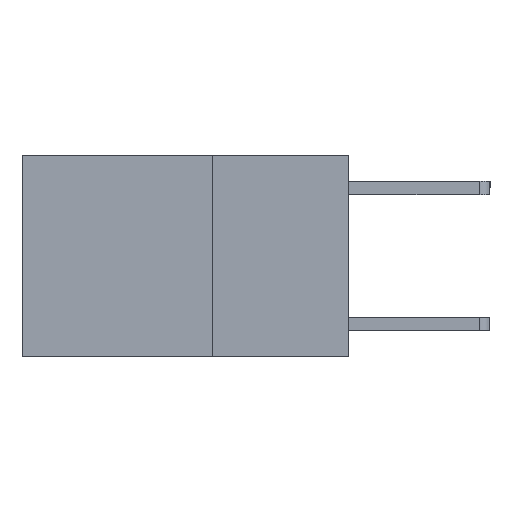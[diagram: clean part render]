
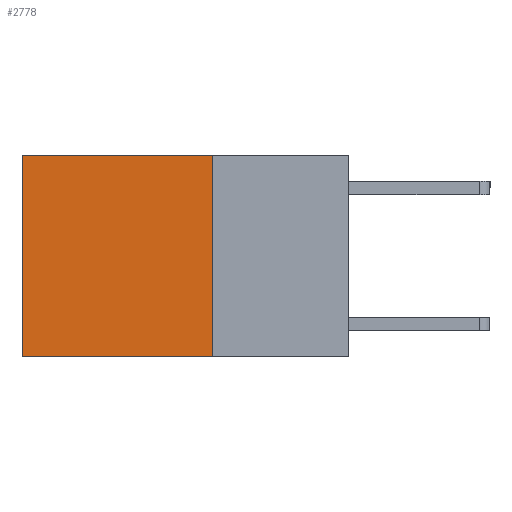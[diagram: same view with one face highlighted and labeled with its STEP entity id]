
A CAD part, left-side view. The second image highlights one B-rep face of the part: STEP entity #2778.
In plain terms, the highlighted planar face has unit normal (-1, 0, 0).
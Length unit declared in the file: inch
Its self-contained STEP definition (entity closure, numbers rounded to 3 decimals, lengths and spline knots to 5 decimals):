
#118 = VECTOR ( 'NONE', #6369, 39.37008 ) ;
#669 = VECTOR ( 'NONE', #2385, 39.37008 ) ;
#998 = AXIS2_PLACEMENT_3D ( 'NONE', #3010, #8167, #5518 ) ;
#1388 = EDGE_LOOP ( 'NONE', ( #7840, #7753, #5368, #7393 ) ) ;
#2066 = CARTESIAN_POINT ( 'NONE',  ( 0.2625, 0.25, 0. ) ) ;
#2385 = DIRECTION ( 'NONE',  ( 0., 1., 0. ) ) ;
#2778 = ADVANCED_FACE ( 'NONE', ( #10967 ), #5635, .F. ) ;
#3010 = CARTESIAN_POINT ( 'NONE',  ( 0.2625, 0.25, 0. ) ) ;
#3142 = EDGE_CURVE ( 'NONE', #8922, #5761, #9167, .T. ) ;
#3333 = EDGE_CURVE ( 'NONE', #9965, #8922, #7741, .T. ) ;
#4451 = EDGE_CURVE ( 'NONE', #8764, #5761, #8564, .T. ) ;
#4697 = CARTESIAN_POINT ( 'NONE',  ( 0.2625, 0.25, 0. ) ) ;
#4727 = CARTESIAN_POINT ( 'NONE',  ( 0.2625, 0.25, -0.37 ) ) ;
#4814 = EDGE_CURVE ( 'NONE', #9965, #8764, #5563, .T. ) ;
#4815 = CARTESIAN_POINT ( 'NONE',  ( 0.2625, 0.6, 0. ) ) ;
#5032 = VECTOR ( 'NONE', #8209, 39.37008 ) ;
#5368 = ORIENTED_EDGE ( 'NONE', *, *, #4814, .F. ) ;
#5393 = CARTESIAN_POINT ( 'NONE',  ( 0.2625, 0.6, 0. ) ) ;
#5518 = DIRECTION ( 'NONE',  ( 0., 0., -1. ) ) ;
#5563 = LINE ( 'NONE', #4697, #5032 ) ;
#5635 = PLANE ( 'NONE',  #998 ) ;
#5761 = VERTEX_POINT ( 'NONE', #9185 ) ;
#6369 = DIRECTION ( 'NONE',  ( 0., 0., -1. ) ) ;
#6824 = CARTESIAN_POINT ( 'NONE',  ( 0.2625, 0.25, 0. ) ) ;
#6982 = VECTOR ( 'NONE', #10303, 39.37008 ) ;
#7393 = ORIENTED_EDGE ( 'NONE', *, *, #3333, .T. ) ;
#7741 = LINE ( 'NONE', #6824, #6982 ) ;
#7753 = ORIENTED_EDGE ( 'NONE', *, *, #4451, .F. ) ;
#7840 = ORIENTED_EDGE ( 'NONE', *, *, #3142, .T. ) ;
#8167 = DIRECTION ( 'NONE',  ( 1., 0., 0. ) ) ;
#8209 = DIRECTION ( 'NONE',  ( 0., 0., -1. ) ) ;
#8564 = LINE ( 'NONE', #9529, #669 ) ;
#8764 = VERTEX_POINT ( 'NONE', #4727 ) ;
#8922 = VERTEX_POINT ( 'NONE', #5393 ) ;
#9167 = LINE ( 'NONE', #4815, #118 ) ;
#9185 = CARTESIAN_POINT ( 'NONE',  ( 0.2625, 0.6, -0.37 ) ) ;
#9529 = CARTESIAN_POINT ( 'NONE',  ( 0.2625, 0.25, -0.37 ) ) ;
#9965 = VERTEX_POINT ( 'NONE', #2066 ) ;
#10303 = DIRECTION ( 'NONE',  ( 0., 1., 0. ) ) ;
#10967 = FACE_OUTER_BOUND ( 'NONE', #1388, .T. ) ;
